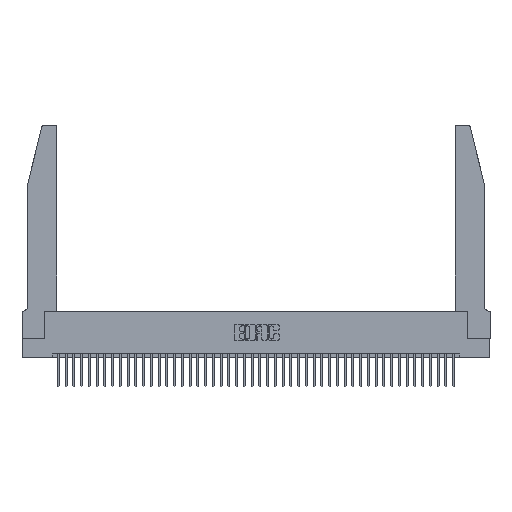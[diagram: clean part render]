
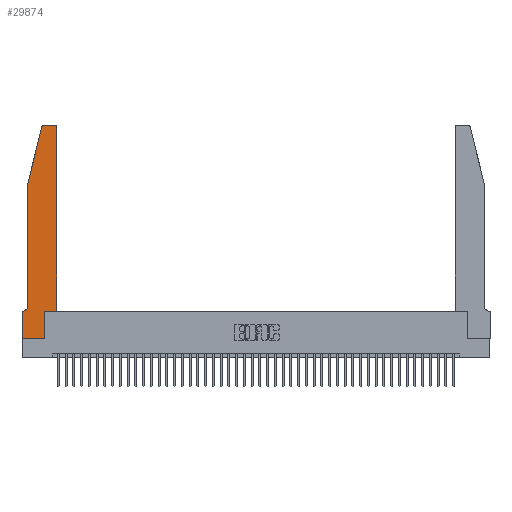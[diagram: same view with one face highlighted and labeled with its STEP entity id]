
A CAD part, top view. The second image highlights one B-rep face of the part: STEP entity #29874.
In plain terms, the highlighted planar face has unit normal (0, 0, 1).
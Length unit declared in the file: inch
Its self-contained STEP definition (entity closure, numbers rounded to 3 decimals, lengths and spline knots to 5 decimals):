
#70 = EDGE_CURVE ( 'NONE', #38245, #41599, #30559, .T. ) ;
#426 = DIRECTION ( 'NONE',  ( 0., 0., 1. ) ) ;
#583 = EDGE_LOOP ( 'NONE', ( #8915, #44199, #1969, #14688, #39354, #3974, #7408, #28567, #22216, #3703, #17847, #9569 ) ) ;
#593 = VERTEX_POINT ( 'NONE', #23627 ) ;
#1588 = CARTESIAN_POINT ( 'NONE',  ( 0.0755, 0.35, 0.37 ) ) ;
#1969 = ORIENTED_EDGE ( 'NONE', *, *, #23008, .T. ) ;
#2302 = DIRECTION ( 'NONE',  ( 0., 0., 1. ) ) ;
#3703 = ORIENTED_EDGE ( 'NONE', *, *, #31078, .T. ) ;
#3974 = ORIENTED_EDGE ( 'NONE', *, *, #37240, .T. ) ;
#4357 = VERTEX_POINT ( 'NONE', #42503 ) ;
#4940 = CARTESIAN_POINT ( 'NONE',  ( 0., 0.35, 0.37 ) ) ;
#5117 = DIRECTION ( 'NONE',  ( 0., 1., 0. ) ) ;
#5190 = LINE ( 'NONE', #35942, #14370 ) ;
#5732 = CARTESIAN_POINT ( 'NONE',  ( 0.0755, 2., 0.37 ) ) ;
#5838 = VECTOR ( 'NONE', #23293, 39.37008 ) ;
#5977 = VECTOR ( 'NONE', #26384, 39.37008 ) ;
#6546 = LINE ( 'NONE', #5732, #14605 ) ;
#6819 = VERTEX_POINT ( 'NONE', #12682 ) ;
#7053 = AXIS2_PLACEMENT_3D ( 'NONE', #21093, #426, #24542 ) ;
#7070 = DIRECTION ( 'NONE',  ( 0., -1., 0. ) ) ;
#7106 = CIRCLE ( 'NONE', #28051, 0.03 ) ;
#7408 = ORIENTED_EDGE ( 'NONE', *, *, #70, .T. ) ;
#8111 = CARTESIAN_POINT ( 'NONE',  ( 0.0055, 0.42, 0.37 ) ) ;
#8853 = EDGE_CURVE ( 'NONE', #593, #6819, #23077, .T. ) ;
#8915 = ORIENTED_EDGE ( 'NONE', *, *, #8853, .T. ) ;
#9569 = ORIENTED_EDGE ( 'NONE', *, *, #27697, .T. ) ;
#9765 = VERTEX_POINT ( 'NONE', #38877 ) ;
#9910 = VERTEX_POINT ( 'NONE', #36353 ) ;
#10471 = EDGE_CURVE ( 'NONE', #20444, #30711, #21014, .T. ) ;
#11574 = DIRECTION ( 'NONE',  ( -1., 0., 0. ) ) ;
#11796 = VECTOR ( 'NONE', #18638, 39.37008 ) ;
#11867 = PLANE ( 'NONE',  #22702 ) ;
#12039 = VERTEX_POINT ( 'NONE', #42311 ) ;
#12256 = EDGE_CURVE ( 'NONE', #41599, #16403, #41007, .T. ) ;
#12519 = CARTESIAN_POINT ( 'NONE',  ( 0.4505, 0.35, 0.37 ) ) ;
#12682 = CARTESIAN_POINT ( 'NONE',  ( 0.284, 2.75, 0.37 ) ) ;
#13620 = CARTESIAN_POINT ( 'NONE',  ( 0.2605, 2.75, 0.37 ) ) ;
#14370 = VECTOR ( 'NONE', #5117, 39.37008 ) ;
#14605 = VECTOR ( 'NONE', #26357, 39.37008 ) ;
#14688 = ORIENTED_EDGE ( 'NONE', *, *, #43574, .T. ) ;
#15113 = LINE ( 'NONE', #12519, #5977 ) ;
#15329 = DIRECTION ( 'NONE',  ( 0., 0., 1. ) ) ;
#16403 = VERTEX_POINT ( 'NONE', #16997 ) ;
#16709 = CARTESIAN_POINT ( 'NONE',  ( 0.4505, 0.35, 0.37 ) ) ;
#16997 = CARTESIAN_POINT ( 'NONE',  ( 0.2865, 0., 0.37 ) ) ;
#17847 = ORIENTED_EDGE ( 'NONE', *, *, #10471, .T. ) ;
#18638 = DIRECTION ( 'NONE',  ( 0., 1., 0. ) ) ;
#19331 = VECTOR ( 'NONE', #7070, 39.37008 ) ;
#19767 = CARTESIAN_POINT ( 'NONE',  ( 0., 0., 0.37 ) ) ;
#20444 = VERTEX_POINT ( 'NONE', #16709 ) ;
#20527 = CIRCLE ( 'NONE', #7053, 0.03 ) ;
#21014 = LINE ( 'NONE', #32169, #11796 ) ;
#21093 = CARTESIAN_POINT ( 'NONE',  ( 0.4205, 2.72, 0.37 ) ) ;
#21913 = VECTOR ( 'NONE', #43467, 39.37008 ) ;
#21989 = VECTOR ( 'NONE', #24042, 39.37008 ) ;
#22013 = EDGE_CURVE ( 'NONE', #12039, #9765, #32023, .T. ) ;
#22216 = ORIENTED_EDGE ( 'NONE', *, *, #36624, .T. ) ;
#22702 = AXIS2_PLACEMENT_3D ( 'NONE', #4940, #15329, #39167 ) ;
#22981 = CARTESIAN_POINT ( 'NONE',  ( 0.284, 2.72, 0.37 ) ) ;
#23008 = EDGE_CURVE ( 'NONE', #9910, #4357, #33168, .T. ) ;
#23077 = LINE ( 'NONE', #13620, #21989 ) ;
#23293 = DIRECTION ( 'NONE',  ( -0.239, -0.971, 0. ) ) ;
#23627 = CARTESIAN_POINT ( 'NONE',  ( 0.4205, 2.75, 0.37 ) ) ;
#24042 = DIRECTION ( 'NONE',  ( -1., 0., 0. ) ) ;
#24542 = DIRECTION ( 'NONE',  ( 1., 0., 0. ) ) ;
#26357 = DIRECTION ( 'NONE',  ( 0., -1., 0. ) ) ;
#26384 = DIRECTION ( 'NONE',  ( 1., 0., 0. ) ) ;
#26401 = DIRECTION ( 'NONE',  ( 1., 0., 0. ) ) ;
#26712 = CARTESIAN_POINT ( 'NONE',  ( 0.0755, 2., 0.37 ) ) ;
#26916 = EDGE_CURVE ( 'NONE', #6819, #9910, #7106, .T. ) ;
#27610 = CARTESIAN_POINT ( 'NONE',  ( 0.2865, 0.35, 0.37 ) ) ;
#27697 = EDGE_CURVE ( 'NONE', #30711, #593, #20527, .T. ) ;
#28051 = AXIS2_PLACEMENT_3D ( 'NONE', #22981, #2302, #26401 ) ;
#28508 = AXIS2_PLACEMENT_3D ( 'NONE', #8111, #32076, #11574 ) ;
#28567 = ORIENTED_EDGE ( 'NONE', *, *, #12256, .T. ) ;
#29149 = CARTESIAN_POINT ( 'NONE',  ( 0., 0., 0.37 ) ) ;
#29874 = ADVANCED_FACE ( 'NONE', ( #35456 ), #11867, .T. ) ;
#30559 = LINE ( 'NONE', #41263, #19331 ) ;
#30711 = VERTEX_POINT ( 'NONE', #37797 ) ;
#31078 = EDGE_CURVE ( 'NONE', #42625, #20444, #15113, .T. ) ;
#32023 = CIRCLE ( 'NONE', #28508, 0.07 ) ;
#32076 = DIRECTION ( 'NONE',  ( 0., 0., -1. ) ) ;
#32169 = CARTESIAN_POINT ( 'NONE',  ( 0.4505, 0.35, 0.37 ) ) ;
#33168 = LINE ( 'NONE', #26712, #5838 ) ;
#35456 = FACE_OUTER_BOUND ( 'NONE', #583, .T. ) ;
#35942 = CARTESIAN_POINT ( 'NONE',  ( 0.2865, 0.35, 0.37 ) ) ;
#36353 = CARTESIAN_POINT ( 'NONE',  ( 0.25487, 2.72718, 0.37 ) ) ;
#36624 = EDGE_CURVE ( 'NONE', #16403, #42625, #5190, .T. ) ;
#37240 = EDGE_CURVE ( 'NONE', #9765, #38245, #42033, .T. ) ;
#37599 = CARTESIAN_POINT ( 'NONE',  ( 0., 0.35, 0.37 ) ) ;
#37797 = CARTESIAN_POINT ( 'NONE',  ( 0.4505, 2.72, 0.37 ) ) ;
#38245 = VERTEX_POINT ( 'NONE', #37599 ) ;
#38877 = CARTESIAN_POINT ( 'NONE',  ( 0.0055, 0.35, 0.37 ) ) ;
#39167 = DIRECTION ( 'NONE',  ( 1., 0., 0. ) ) ;
#39354 = ORIENTED_EDGE ( 'NONE', *, *, #22013, .T. ) ;
#40975 = VECTOR ( 'NONE', #42551, 39.37008 ) ;
#41007 = LINE ( 'NONE', #19767, #21913 ) ;
#41263 = CARTESIAN_POINT ( 'NONE',  ( 0., 0., 0.37 ) ) ;
#41599 = VERTEX_POINT ( 'NONE', #29149 ) ;
#42033 = LINE ( 'NONE', #1588, #40975 ) ;
#42311 = CARTESIAN_POINT ( 'NONE',  ( 0.0755, 0.42, 0.37 ) ) ;
#42503 = CARTESIAN_POINT ( 'NONE',  ( 0.0755, 2., 0.37 ) ) ;
#42551 = DIRECTION ( 'NONE',  ( -1., 0., 0. ) ) ;
#42625 = VERTEX_POINT ( 'NONE', #27610 ) ;
#43467 = DIRECTION ( 'NONE',  ( 1., 0., 0. ) ) ;
#43574 = EDGE_CURVE ( 'NONE', #4357, #12039, #6546, .T. ) ;
#44199 = ORIENTED_EDGE ( 'NONE', *, *, #26916, .T. ) ;
